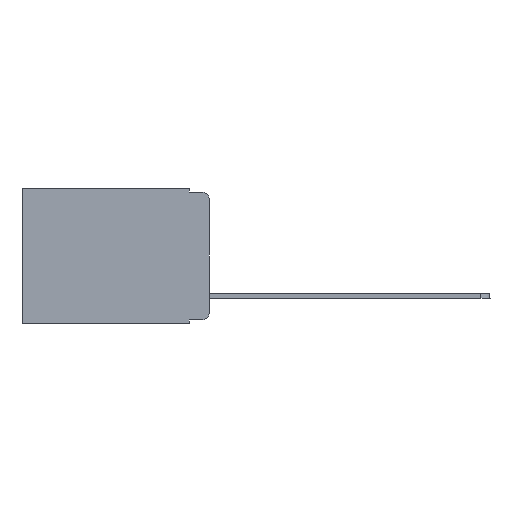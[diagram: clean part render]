
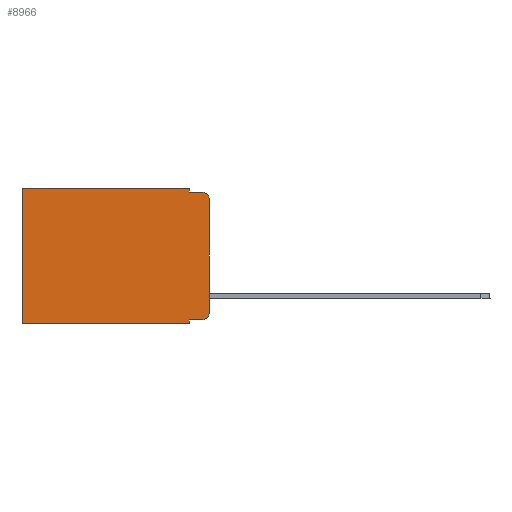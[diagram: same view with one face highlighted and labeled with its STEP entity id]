
A CAD part, left-side view. The second image highlights one B-rep face of the part: STEP entity #8966.
In plain terms, the highlighted planar face has unit normal (-1, 0, 0).
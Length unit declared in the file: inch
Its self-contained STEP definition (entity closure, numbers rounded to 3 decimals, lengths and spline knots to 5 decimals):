
#136 = DIRECTION ( 'NONE',  ( 0., 0., -1. ) ) ;
#451 = LINE ( 'NONE', #22925, #18957 ) ;
#768 = VERTEX_POINT ( 'NONE', #8312 ) ;
#1032 = EDGE_CURVE ( 'NONE', #768, #3126, #4278, .T. ) ;
#1177 = DIRECTION ( 'NONE',  ( 0., 0., -1. ) ) ;
#1463 = DIRECTION ( 'NONE',  ( 0., 1., 0. ) ) ;
#1513 = CARTESIAN_POINT ( 'NONE',  ( 0.298, 0.051, 0. ) ) ;
#1919 = CARTESIAN_POINT ( 'NONE',  ( 0.298, 0., 0. ) ) ;
#2446 = CARTESIAN_POINT ( 'NONE',  ( 0.298, 0.02, -0.313 ) ) ;
#2941 = CARTESIAN_POINT ( 'NONE',  ( 0.298, 0.473, 0. ) ) ;
#3126 = VERTEX_POINT ( 'NONE', #19501 ) ;
#4167 = DIRECTION ( 'NONE',  ( 0., 0., -1. ) ) ;
#4278 = LINE ( 'NONE', #14287, #19721 ) ;
#4520 = VERTEX_POINT ( 'NONE', #18388 ) ;
#4627 = EDGE_LOOP ( 'NONE', ( #14270, #18445, #13889, #22480, #20715, #21030, #21996, #14923, #16366, #5773 ) ) ;
#4916 = FACE_OUTER_BOUND ( 'NONE', #4627, .T. ) ;
#4971 = VECTOR ( 'NONE', #5383, 39.37008 ) ;
#5029 = CARTESIAN_POINT ( 'NONE',  ( 0.298, 0., 0. ) ) ;
#5299 = CIRCLE ( 'NONE', #15726, 0.02 ) ;
#5383 = DIRECTION ( 'NONE',  ( 0., -1., 0. ) ) ;
#5773 = ORIENTED_EDGE ( 'NONE', *, *, #16113, .T. ) ;
#5952 = DIRECTION ( 'NONE',  ( -1., 0., 0. ) ) ;
#6434 = AXIS2_PLACEMENT_3D ( 'NONE', #22092, #5952, #4167 ) ;
#6621 = CARTESIAN_POINT ( 'NONE',  ( 0.298, 0.051, -0.01 ) ) ;
#7496 = CARTESIAN_POINT ( 'NONE',  ( 0.298, 0.051, -0.343 ) ) ;
#8312 = CARTESIAN_POINT ( 'NONE',  ( 0.298, 0.051, 0. ) ) ;
#8405 = LINE ( 'NONE', #19756, #10346 ) ;
#8575 = VERTEX_POINT ( 'NONE', #13422 ) ;
#8635 = LINE ( 'NONE', #14299, #4971 ) ;
#8705 = DIRECTION ( 'NONE',  ( 0., 0., -1. ) ) ;
#8757 = DIRECTION ( 'NONE',  ( 0., 0., -1. ) ) ;
#8966 = ADVANCED_FACE ( 'NONE', ( #4916 ), #10839, .F. ) ;
#9169 = EDGE_CURVE ( 'NONE', #17334, #8575, #19212, .T. ) ;
#9734 = DIRECTION ( 'NONE',  ( 0., -1., 0. ) ) ;
#10346 = VECTOR ( 'NONE', #136, 39.37008 ) ;
#10462 = CARTESIAN_POINT ( 'NONE',  ( 0.298, 0.051, -0.333 ) ) ;
#10839 = PLANE ( 'NONE',  #14038 ) ;
#11058 = LINE ( 'NONE', #2941, #21988 ) ;
#11269 = EDGE_CURVE ( 'NONE', #14438, #13797, #8635, .T. ) ;
#11908 = DIRECTION ( 'NONE',  ( -1., 0., 0. ) ) ;
#12289 = CIRCLE ( 'NONE', #6434, 0.02 ) ;
#12374 = DIRECTION ( 'NONE',  ( 0., 0., -1. ) ) ;
#12385 = LINE ( 'NONE', #5029, #15194 ) ;
#13246 = EDGE_CURVE ( 'NONE', #3126, #17255, #11058, .T. ) ;
#13282 = VECTOR ( 'NONE', #9734, 39.37008 ) ;
#13422 = CARTESIAN_POINT ( 'NONE',  ( 0.298, 0.02, -0.01 ) ) ;
#13797 = VERTEX_POINT ( 'NONE', #16168 ) ;
#13889 = ORIENTED_EDGE ( 'NONE', *, *, #9169, .F. ) ;
#14038 = AXIS2_PLACEMENT_3D ( 'NONE', #1919, #14414, #8757 ) ;
#14270 = ORIENTED_EDGE ( 'NONE', *, *, #14519, .F. ) ;
#14287 = CARTESIAN_POINT ( 'NONE',  ( 0.298, 0., 0. ) ) ;
#14299 = CARTESIAN_POINT ( 'NONE',  ( 0.298, 0.051, -0.333 ) ) ;
#14414 = DIRECTION ( 'NONE',  ( 1., 0., 0. ) ) ;
#14438 = VERTEX_POINT ( 'NONE', #10462 ) ;
#14519 = EDGE_CURVE ( 'NONE', #4520, #18348, #12385, .T. ) ;
#14923 = ORIENTED_EDGE ( 'NONE', *, *, #17470, .F. ) ;
#15194 = VECTOR ( 'NONE', #12374, 39.37008 ) ;
#15726 = AXIS2_PLACEMENT_3D ( 'NONE', #2446, #11908, #8705 ) ;
#16113 = EDGE_CURVE ( 'NONE', #13797, #18348, #5299, .T. ) ;
#16168 = CARTESIAN_POINT ( 'NONE',  ( 0.298, 0.02, -0.333 ) ) ;
#16366 = ORIENTED_EDGE ( 'NONE', *, *, #11269, .T. ) ;
#17113 = VERTEX_POINT ( 'NONE', #7496 ) ;
#17255 = VERTEX_POINT ( 'NONE', #19232 ) ;
#17334 = VERTEX_POINT ( 'NONE', #6621 ) ;
#17470 = EDGE_CURVE ( 'NONE', #14438, #17113, #20192, .T. ) ;
#17735 = EDGE_CURVE ( 'NONE', #4520, #8575, #12289, .T. ) ;
#17903 = DIRECTION ( 'NONE',  ( 0., 1., 0. ) ) ;
#18196 = EDGE_CURVE ( 'NONE', #768, #17334, #8405, .T. ) ;
#18348 = VERTEX_POINT ( 'NONE', #18694 ) ;
#18388 = CARTESIAN_POINT ( 'NONE',  ( 0.298, 0., -0.03 ) ) ;
#18445 = ORIENTED_EDGE ( 'NONE', *, *, #17735, .T. ) ;
#18694 = CARTESIAN_POINT ( 'NONE',  ( 0.298, 0., -0.313 ) ) ;
#18957 = VECTOR ( 'NONE', #1463, 39.37008 ) ;
#19212 = LINE ( 'NONE', #20478, #13282 ) ;
#19232 = CARTESIAN_POINT ( 'NONE',  ( 0.298, 0.473, -0.343 ) ) ;
#19386 = DIRECTION ( 'NONE',  ( 0., 0., -1. ) ) ;
#19501 = CARTESIAN_POINT ( 'NONE',  ( 0.298, 0.473, 0. ) ) ;
#19653 = EDGE_CURVE ( 'NONE', #17113, #17255, #451, .T. ) ;
#19721 = VECTOR ( 'NONE', #17903, 39.37008 ) ;
#19756 = CARTESIAN_POINT ( 'NONE',  ( 0.298, 0.051, 0. ) ) ;
#20192 = LINE ( 'NONE', #1513, #21039 ) ;
#20478 = CARTESIAN_POINT ( 'NONE',  ( 0.298, 0.051, -0.01 ) ) ;
#20715 = ORIENTED_EDGE ( 'NONE', *, *, #1032, .T. ) ;
#21030 = ORIENTED_EDGE ( 'NONE', *, *, #13246, .T. ) ;
#21039 = VECTOR ( 'NONE', #19386, 39.37008 ) ;
#21988 = VECTOR ( 'NONE', #1177, 39.37008 ) ;
#21996 = ORIENTED_EDGE ( 'NONE', *, *, #19653, .F. ) ;
#22092 = CARTESIAN_POINT ( 'NONE',  ( 0.298, 0.02, -0.03 ) ) ;
#22480 = ORIENTED_EDGE ( 'NONE', *, *, #18196, .F. ) ;
#22925 = CARTESIAN_POINT ( 'NONE',  ( 0.298, 0., -0.343 ) ) ;
